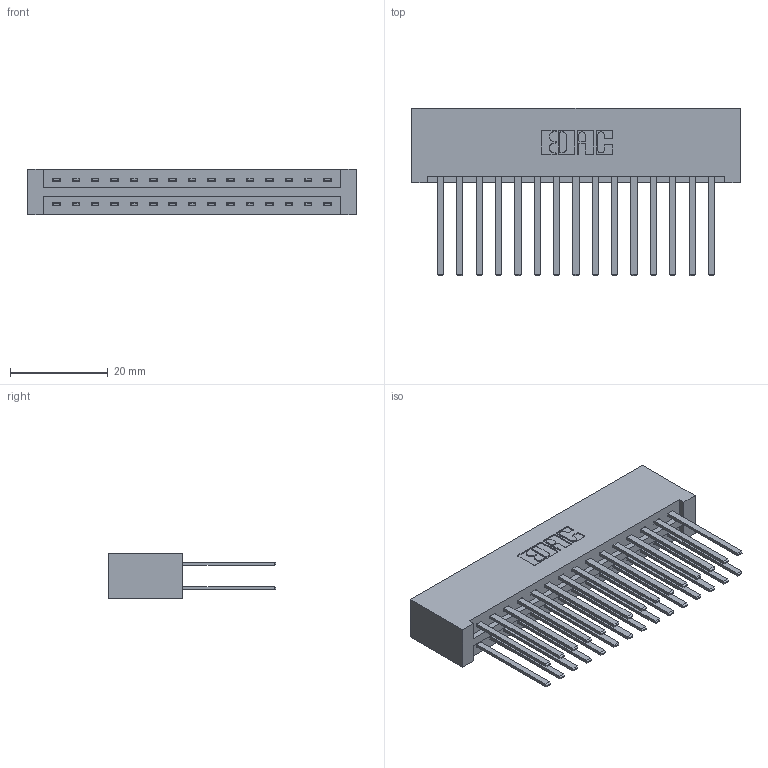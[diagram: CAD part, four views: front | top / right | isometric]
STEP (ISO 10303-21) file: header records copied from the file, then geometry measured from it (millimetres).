
FILE_DESCRIPTION (( 'STEP AP203' ), '1' );
FILE_NAME ('387-030-544-201.STEP', '2019-10-17T14:41:55', ( '' ), ( '' ), 'SwSTEP 2.0', 'SolidWorks 2016', '' );
FILE_SCHEMA (( 'CONFIG_CONTROL_DESIGN' ));
Length unit declared in the file: inch
Products named in the file (3): 345-292-001_345-293-144; 387-030-544-201; 337 Part_No Mounting Lugs
Assembly tree (31 placements, depth 2):
  387-030-544-201
    337 Part_No Mounting Lugs
    345-292-001_345-293-144  x30
Bounding box: 67.31 x 34.3 x 9.4 mm (x, y, z)
Volume: 7915.5 mm3; surface area: 10116.2 mm2
Topology: 31 solids, 31 shells, 1546 faces, 4577 edges, 3010 vertices
Faces by surface type: plane 1086, cylinder 460
Entity records: 14661 total; most frequent: CARTESIAN_POINT 2490, ORIENTED_EDGE 2426, DIRECTION 2157, EDGE_CURVE 1213, LINE 1097, VECTOR 1097, VERTEX_POINT 806, AXIS2_PLACEMENT_3D 530
